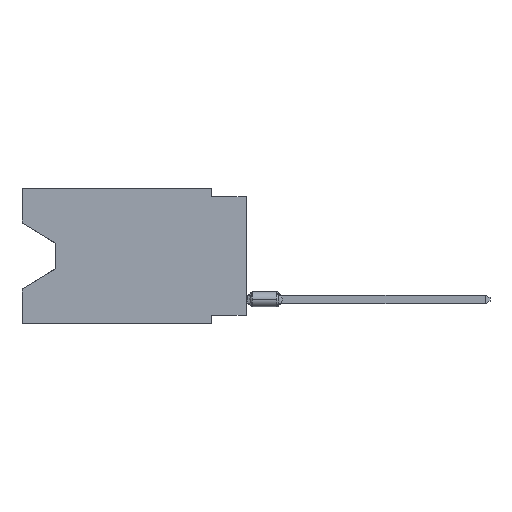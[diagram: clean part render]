
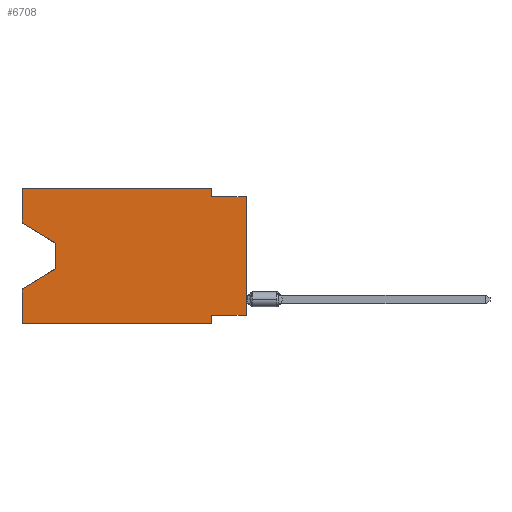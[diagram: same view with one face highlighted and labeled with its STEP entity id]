
A CAD part, left-side view. The second image highlights one B-rep face of the part: STEP entity #6708.
In plain terms, the highlighted planar face has unit normal (-1, 0, 0).
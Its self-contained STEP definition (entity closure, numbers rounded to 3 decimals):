
#461 = DIRECTION ( 'NONE',  ( 0., 1., 0. ) ) ;
#651 = LINE ( 'NONE', #4771, #3869 ) ;
#900 = DIRECTION ( 'NONE',  ( 0., 0., 1. ) ) ;
#1161 = VECTOR ( 'NONE', #7461, 1000. ) ;
#1211 = CARTESIAN_POINT ( 'NONE',  ( 0., 2.54, -9.271 ) ) ;
#1621 = DIRECTION ( 'NONE',  ( 0., 0., -1. ) ) ;
#1716 = FACE_OUTER_BOUND ( 'NONE', #2149, .T. ) ;
#1736 = CARTESIAN_POINT ( 'NONE',  ( 0., 2.54, -9.906 ) ) ;
#1907 = LINE ( 'NONE', #15943, #11863 ) ;
#2018 = LINE ( 'NONE', #16047, #4140 ) ;
#2085 = EDGE_CURVE ( 'NONE', #3539, #16217, #13620, .T. ) ;
#2149 = EDGE_LOOP ( 'NONE', ( #11581, #13322, #3234, #3735, #15266, #11977, #11923, #14328, #2279, #3992, #10113, #7335 ) ) ;
#2168 = DIRECTION ( 'NONE',  ( 0., 0., 1. ) ) ;
#2279 = ORIENTED_EDGE ( 'NONE', *, *, #9011, .F. ) ;
#2319 = CARTESIAN_POINT ( 'NONE',  ( 0., 13.97, -4.013 ) ) ;
#3169 = LINE ( 'NONE', #13589, #15062 ) ;
#3234 = ORIENTED_EDGE ( 'NONE', *, *, #4237, .T. ) ;
#3430 = CARTESIAN_POINT ( 'NONE',  ( 0., 2.54, -9.906 ) ) ;
#3481 = AXIS2_PLACEMENT_3D ( 'NONE', #12063, #14622, #1621 ) ;
#3530 = DIRECTION ( 'NONE',  ( 0., 0., 1. ) ) ;
#3539 = VERTEX_POINT ( 'NONE', #1211 ) ;
#3635 = VERTEX_POINT ( 'NONE', #8931 ) ;
#3735 = ORIENTED_EDGE ( 'NONE', *, *, #16767, .F. ) ;
#3739 = VERTEX_POINT ( 'NONE', #9360 ) ;
#3867 = VECTOR ( 'NONE', #12172, 1000. ) ;
#3869 = VECTOR ( 'NONE', #900, 1000. ) ;
#3992 = ORIENTED_EDGE ( 'NONE', *, *, #4751, .F. ) ;
#4140 = VECTOR ( 'NONE', #10926, 1000. ) ;
#4237 = EDGE_CURVE ( 'NONE', #12184, #6144, #2018, .T. ) ;
#4259 = CARTESIAN_POINT ( 'NONE',  ( 0., 16.383, -9.906 ) ) ;
#4460 = CARTESIAN_POINT ( 'NONE',  ( 0., 16.383, -2.546 ) ) ;
#4751 = EDGE_CURVE ( 'NONE', #3739, #12192, #16622, .T. ) ;
#4771 = CARTESIAN_POINT ( 'NONE',  ( 0., 16.383, 0. ) ) ;
#4813 = DIRECTION ( 'NONE',  ( 0., 0., -1. ) ) ;
#4984 = LINE ( 'NONE', #6027, #1161 ) ;
#5090 = CARTESIAN_POINT ( 'NONE',  ( 0., 16.383, -7.36 ) ) ;
#5464 = EDGE_CURVE ( 'NONE', #16166, #12184, #13009, .T. ) ;
#5619 = CARTESIAN_POINT ( 'NONE',  ( 0., 16.383, -9.906 ) ) ;
#5744 = VERTEX_POINT ( 'NONE', #11756 ) ;
#5805 = EDGE_CURVE ( 'NONE', #16852, #16217, #12356, .T. ) ;
#5964 = LINE ( 'NONE', #6216, #13298 ) ;
#6011 = EDGE_CURVE ( 'NONE', #13272, #3635, #5964, .T. ) ;
#6027 = CARTESIAN_POINT ( 'NONE',  ( 0., 16.383, 0. ) ) ;
#6144 = VERTEX_POINT ( 'NONE', #5090 ) ;
#6213 = VECTOR ( 'NONE', #4813, 1000. ) ;
#6216 = CARTESIAN_POINT ( 'NONE',  ( 0., 16.383, 0. ) ) ;
#6708 = ADVANCED_FACE ( 'NONE', ( #1716 ), #16159, .F. ) ;
#6843 = CARTESIAN_POINT ( 'NONE',  ( 0., 0., -9.271 ) ) ;
#7335 = ORIENTED_EDGE ( 'NONE', *, *, #6011, .F. ) ;
#7452 = CARTESIAN_POINT ( 'NONE',  ( 0., 13.97, -4.013 ) ) ;
#7461 = DIRECTION ( 'NONE',  ( 0., -1., 0. ) ) ;
#7489 = CARTESIAN_POINT ( 'NONE',  ( 0., 2.54, 0. ) ) ;
#8382 = DIRECTION ( 'NONE',  ( 0., -0.855, -0.519 ) ) ;
#8646 = EDGE_CURVE ( 'NONE', #13290, #3539, #1907, .T. ) ;
#8681 = LINE ( 'NONE', #13813, #8766 ) ;
#8766 = VECTOR ( 'NONE', #2168, 1000. ) ;
#8931 = CARTESIAN_POINT ( 'NONE',  ( 0., 16.383, 0. ) ) ;
#9011 = EDGE_CURVE ( 'NONE', #12192, #5744, #3169, .T. ) ;
#9360 = CARTESIAN_POINT ( 'NONE',  ( 0., 2.54, 0. ) ) ;
#9408 = CARTESIAN_POINT ( 'NONE',  ( 0., 16.383, -2.546 ) ) ;
#9610 = VECTOR ( 'NONE', #11407, 1000. ) ;
#9689 = CARTESIAN_POINT ( 'NONE',  ( 0., 13.97, -5.893 ) ) ;
#10113 = ORIENTED_EDGE ( 'NONE', *, *, #10893, .F. ) ;
#10442 = VECTOR ( 'NONE', #8382, 1000. ) ;
#10893 = EDGE_CURVE ( 'NONE', #3635, #3739, #4984, .T. ) ;
#10926 = DIRECTION ( 'NONE',  ( 0., 0.855, -0.519 ) ) ;
#11407 = DIRECTION ( 'NONE',  ( 0., 0., -1. ) ) ;
#11581 = ORIENTED_EDGE ( 'NONE', *, *, #16424, .T. ) ;
#11756 = CARTESIAN_POINT ( 'NONE',  ( 0., 0., -0.635 ) ) ;
#11863 = VECTOR ( 'NONE', #461, 1000. ) ;
#11923 = ORIENTED_EDGE ( 'NONE', *, *, #8646, .F. ) ;
#11977 = ORIENTED_EDGE ( 'NONE', *, *, #2085, .F. ) ;
#12063 = CARTESIAN_POINT ( 'NONE',  ( 0., 16.383, 0. ) ) ;
#12172 = DIRECTION ( 'NONE',  ( 0., 0., -1. ) ) ;
#12184 = VERTEX_POINT ( 'NONE', #9689 ) ;
#12192 = VERTEX_POINT ( 'NONE', #12239 ) ;
#12209 = VECTOR ( 'NONE', #16025, 1000. ) ;
#12239 = CARTESIAN_POINT ( 'NONE',  ( 0., 2.54, -0.635 ) ) ;
#12356 = LINE ( 'NONE', #4259, #12209 ) ;
#13009 = LINE ( 'NONE', #2319, #6213 ) ;
#13272 = VERTEX_POINT ( 'NONE', #9408 ) ;
#13290 = VERTEX_POINT ( 'NONE', #6843 ) ;
#13298 = VECTOR ( 'NONE', #3530, 1000. ) ;
#13322 = ORIENTED_EDGE ( 'NONE', *, *, #5464, .T. ) ;
#13589 = CARTESIAN_POINT ( 'NONE',  ( 0., 0., -0.635 ) ) ;
#13620 = LINE ( 'NONE', #1736, #3867 ) ;
#13813 = CARTESIAN_POINT ( 'NONE',  ( 0., 0., 0. ) ) ;
#14328 = ORIENTED_EDGE ( 'NONE', *, *, #16726, .T. ) ;
#14622 = DIRECTION ( 'NONE',  ( 1., 0., 0. ) ) ;
#14957 = LINE ( 'NONE', #4460, #10442 ) ;
#15062 = VECTOR ( 'NONE', #16245, 1000. ) ;
#15266 = ORIENTED_EDGE ( 'NONE', *, *, #5805, .T. ) ;
#15943 = CARTESIAN_POINT ( 'NONE',  ( 0., 0., -9.271 ) ) ;
#16025 = DIRECTION ( 'NONE',  ( 0., -1., 0. ) ) ;
#16047 = CARTESIAN_POINT ( 'NONE',  ( 0., 13.97, -5.893 ) ) ;
#16159 = PLANE ( 'NONE',  #3481 ) ;
#16166 = VERTEX_POINT ( 'NONE', #7452 ) ;
#16217 = VERTEX_POINT ( 'NONE', #3430 ) ;
#16245 = DIRECTION ( 'NONE',  ( 0., -1., 0. ) ) ;
#16424 = EDGE_CURVE ( 'NONE', #13272, #16166, #14957, .T. ) ;
#16622 = LINE ( 'NONE', #7489, #9610 ) ;
#16726 = EDGE_CURVE ( 'NONE', #13290, #5744, #8681, .T. ) ;
#16767 = EDGE_CURVE ( 'NONE', #16852, #6144, #651, .T. ) ;
#16852 = VERTEX_POINT ( 'NONE', #5619 ) ;
